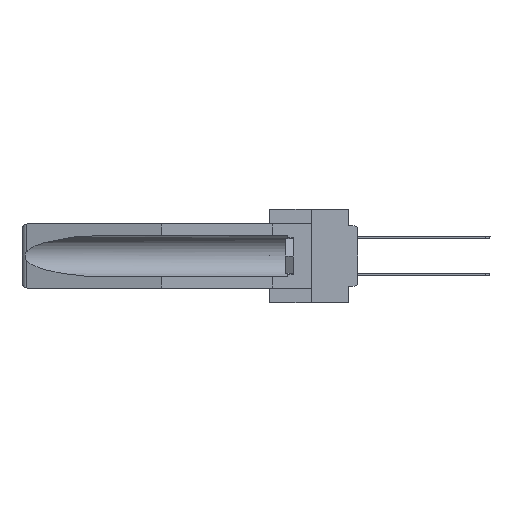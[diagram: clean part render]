
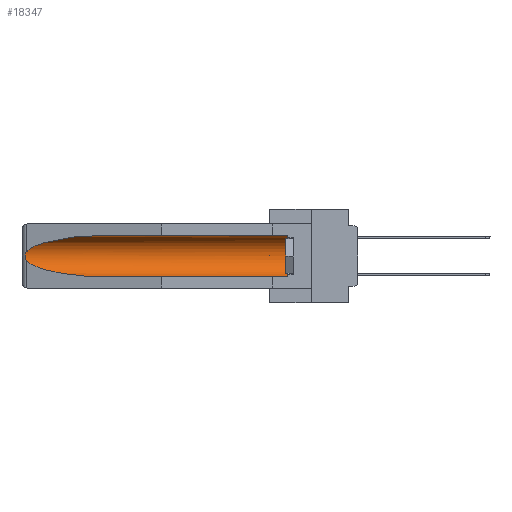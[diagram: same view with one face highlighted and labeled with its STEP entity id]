
A CAD part, left-side view. The second image highlights one B-rep face of the part: STEP entity #18347.
In plain terms, the highlighted cylindrical face has radius 2.857 mm (diameter 5.715 mm), a partial arc.
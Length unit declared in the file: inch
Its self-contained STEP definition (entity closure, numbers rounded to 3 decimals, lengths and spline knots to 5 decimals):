
#715 = EDGE_CURVE ( 'NONE', #32056, #30088, #17128, .T. ) ;
#1768 = CARTESIAN_POINT ( 'NONE',  ( 0.26537, 1.52718, -0.19328 ) ) ;
#3240 =( BOUNDED_CURVE ( )  B_SPLINE_CURVE ( 3, ( #11420, #20311, #32587, #39050 ),
 .UNSPECIFIED., .F., .F. ) 
 B_SPLINE_CURVE_WITH_KNOTS ( ( 4, 4 ),
 ( 0.1948, 1.5708 ),
 .UNSPECIFIED. ) 
 CURVE ( )  GEOMETRIC_REPRESENTATION_ITEM ( )  RATIONAL_B_SPLINE_CURVE ( ( 1., 0.848, 0.848, 1. ) ) 
 REPRESENTATION_ITEM ( '' )  );
#4415 = AXIS2_PLACEMENT_3D ( 'NONE', #36986, #18230, #12360 ) ;
#4467 = DIRECTION ( 'NONE',  ( 0., -1., 0. ) ) ;
#4560 = CARTESIAN_POINT ( 'NONE',  ( 0.155, 0.126, -0.059 ) ) ;
#4775 = CARTESIAN_POINT ( 'NONE',  ( 0.2673, 1.53269, -0.17917 ) ) ;
#5380 = CARTESIAN_POINT ( 'NONE',  ( 0.2675, 1.53308, -0.16763 ) ) ;
#5576 = CARTESIAN_POINT ( 'NONE',  ( 0.26537, 1.52718, -0.14972 ) ) ;
#6677 = DIRECTION ( 'NONE',  ( 0., 0., 1. ) ) ;
#7795 = EDGE_CURVE ( 'NONE', #12089, #35230, #18430, .T. ) ;
#9224 = LINE ( 'NONE', #17922, #29403 ) ;
#9430 = DIRECTION ( 'NONE',  ( 0., 1., 0. ) ) ;
#10900 = ORIENTED_EDGE ( 'NONE', *, *, #20741, .T. ) ;
#11420 = CARTESIAN_POINT ( 'NONE',  ( 0.26537, 1.52718, -0.19328 ) ) ;
#11823 = CARTESIAN_POINT ( 'NONE',  ( 0.2673, 1.5327, -0.16383 ) ) ;
#11981 = CYLINDRICAL_SURFACE ( 'NONE', #4415, 0.1125 ) ;
#12089 = VERTEX_POINT ( 'NONE', #13761 ) ;
#12360 = DIRECTION ( 'NONE',  ( 0., 0., 1. ) ) ;
#13761 = CARTESIAN_POINT ( 'NONE',  ( 0.155, 0.126, -0.284 ) ) ;
#13834 = B_SPLINE_CURVE_WITH_KNOTS ( 'NONE', 3,
 ( #5576, #14849, #38648, #11823, #5380, #20108, #4775, #17084, #29368, #1768 ),
 .UNSPECIFIED., .F., .F.,
 ( 4, 2, 2, 2, 4 ),
 ( 0., 0.00029, 0.00058, 0.00087, 0.00117 ),
 .UNSPECIFIED. ) ;
#14849 = CARTESIAN_POINT ( 'NONE',  ( 0.26597, 1.52961, -0.15275 ) ) ;
#15703 = VECTOR ( 'NONE', #30664, 39.37008 ) ;
#17084 = CARTESIAN_POINT ( 'NONE',  ( 0.26655, 1.53094, -0.18657 ) ) ;
#17128 =( BOUNDED_CURVE ( )  B_SPLINE_CURVE ( 3, ( #36374, #36576, #21069, #24304 ),
 .UNSPECIFIED., .F., .F. ) 
 B_SPLINE_CURVE_WITH_KNOTS ( ( 4, 4 ),
 ( 4.71239, 6.08839 ),
 .UNSPECIFIED. ) 
 CURVE ( )  GEOMETRIC_REPRESENTATION_ITEM ( )  RATIONAL_B_SPLINE_CURVE ( ( 1., 0.848, 0.848, 1. ) ) 
 REPRESENTATION_ITEM ( '' )  );
#17922 = CARTESIAN_POINT ( 'NONE',  ( 0.155, -0.30754, -0.284 ) ) ;
#17945 = EDGE_LOOP ( 'NONE', ( #28438, #10900, #22836, #24896, #20398, #21038 ) ) ;
#18230 = DIRECTION ( 'NONE',  ( 0., 1., 0. ) ) ;
#18347 = ADVANCED_FACE ( 'NONE', ( #27134 ), #11981, .F. ) ;
#18430 = CIRCLE ( 'NONE', #39664, 0.1125 ) ;
#20108 = CARTESIAN_POINT ( 'NONE',  ( 0.2675, 1.53308, -0.17534 ) ) ;
#20311 = CARTESIAN_POINT ( 'NONE',  ( 0.25451, 1.48313, -0.24835 ) ) ;
#20398 = ORIENTED_EDGE ( 'NONE', *, *, #7795, .T. ) ;
#20741 = EDGE_CURVE ( 'NONE', #30088, #29941, #13834, .T. ) ;
#20766 = EDGE_CURVE ( 'NONE', #29941, #38785, #3240, .T. ) ;
#21038 = ORIENTED_EDGE ( 'NONE', *, *, #33015, .T. ) ;
#21069 = CARTESIAN_POINT ( 'NONE',  ( 0.25451, 1.48313, -0.09465 ) ) ;
#22836 = ORIENTED_EDGE ( 'NONE', *, *, #20766, .T. ) ;
#23604 = EDGE_CURVE ( 'NONE', #12089, #38785, #9224, .T. ) ;
#24304 = CARTESIAN_POINT ( 'NONE',  ( 0.26537, 1.52718, -0.14972 ) ) ;
#24896 = ORIENTED_EDGE ( 'NONE', *, *, #23604, .F. ) ;
#26249 = CARTESIAN_POINT ( 'NONE',  ( 0.26537, 1.52718, -0.19328 ) ) ;
#27134 = FACE_OUTER_BOUND ( 'NONE', #17945, .T. ) ;
#28221 = CARTESIAN_POINT ( 'NONE',  ( 0.26537, 1.52718, -0.14972 ) ) ;
#28438 = ORIENTED_EDGE ( 'NONE', *, *, #715, .T. ) ;
#28475 = CARTESIAN_POINT ( 'NONE',  ( 0.155, 0.126, -0.1715 ) ) ;
#29368 = CARTESIAN_POINT ( 'NONE',  ( 0.26597, 1.5296, -0.19026 ) ) ;
#29403 = VECTOR ( 'NONE', #9430, 39.37008 ) ;
#29941 = VERTEX_POINT ( 'NONE', #26249 ) ;
#30088 = VERTEX_POINT ( 'NONE', #28221 ) ;
#30664 = DIRECTION ( 'NONE',  ( 0., 1., 0. ) ) ;
#32056 = VERTEX_POINT ( 'NONE', #39056 ) ;
#32587 = CARTESIAN_POINT ( 'NONE',  ( 0.21114, 1.30732, -0.284 ) ) ;
#33015 = EDGE_CURVE ( 'NONE', #35230, #32056, #39752, .T. ) ;
#35230 = VERTEX_POINT ( 'NONE', #4560 ) ;
#36374 = CARTESIAN_POINT ( 'NONE',  ( 0.155, 1.07973, -0.059 ) ) ;
#36576 = CARTESIAN_POINT ( 'NONE',  ( 0.21114, 1.30732, -0.059 ) ) ;
#36723 = CARTESIAN_POINT ( 'NONE',  ( 0.155, 1.07973, -0.284 ) ) ;
#36743 = CARTESIAN_POINT ( 'NONE',  ( 0.155, -0.30754, -0.059 ) ) ;
#36986 = CARTESIAN_POINT ( 'NONE',  ( 0.155, -0.30754, -0.1715 ) ) ;
#38648 = CARTESIAN_POINT ( 'NONE',  ( 0.26654, 1.53092, -0.15636 ) ) ;
#38785 = VERTEX_POINT ( 'NONE', #36723 ) ;
#39050 = CARTESIAN_POINT ( 'NONE',  ( 0.155, 1.07973, -0.284 ) ) ;
#39056 = CARTESIAN_POINT ( 'NONE',  ( 0.155, 1.07973, -0.059 ) ) ;
#39664 = AXIS2_PLACEMENT_3D ( 'NONE', #28475, #4467, #6677 ) ;
#39752 = LINE ( 'NONE', #36743, #15703 ) ;
